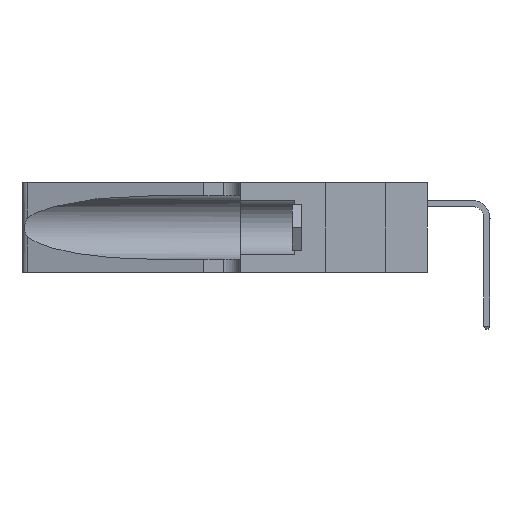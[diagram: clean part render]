
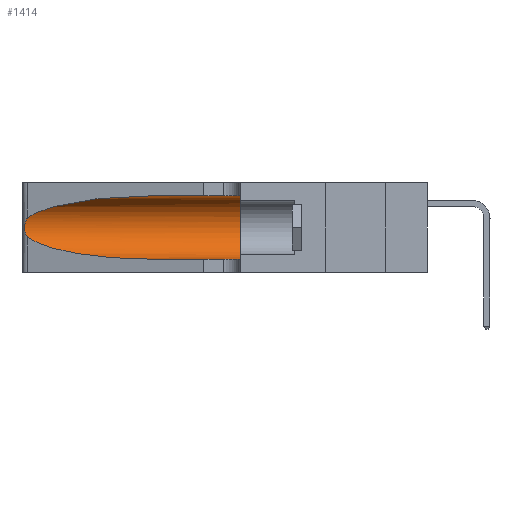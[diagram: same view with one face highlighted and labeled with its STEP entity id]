
A CAD part, left-side view. The second image highlights one B-rep face of the part: STEP entity #1414.
In plain terms, the highlighted cylindrical face has radius 3.308 mm (diameter 6.617 mm), a partial arc.
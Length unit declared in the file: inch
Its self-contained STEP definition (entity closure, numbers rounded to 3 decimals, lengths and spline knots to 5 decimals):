
#1414 = ADVANCED_FACE ( 'NONE', ( #6465 ), #5211, .F. ) ;
#1997 = LINE ( 'NONE', #23070, #11360 ) ;
#3071 = CARTESIAN_POINT ( 'NONE',  ( 0.26075, 1.23896, 0.178 ) ) ;
#3637 = ORIENTED_EDGE ( 'NONE', *, *, #45801, .T. ) ;
#5211 = CYLINDRICAL_SURFACE ( 'NONE', #36076, 0.13025 ) ;
#6465 = FACE_OUTER_BOUND ( 'NONE', #14132, .T. ) ;
#6908 = CARTESIAN_POINT ( 'NONE',  ( 0.25555, 1.22994, 0.2215 ) ) ;
#7047 = EDGE_CURVE ( 'NONE', #12578, #18360, #1997, .T. ) ;
#7082 = CARTESIAN_POINT ( 'NONE',  ( 0.25856, 1.23593, 0.16098 ) ) ;
#8322 = VERTEX_POINT ( 'NONE', #33236 ) ;
#9508 = CARTESIAN_POINT ( 'NONE',  ( 0.1305, 0.72297, 0.05475 ) ) ;
#10535 = CARTESIAN_POINT ( 'NONE',  ( 0.25487, 1.22718, 0.14631 ) ) ;
#11056 = CARTESIAN_POINT ( 'NONE',  ( 0.25639, 1.23186, 0.15144 ) ) ;
#11360 = VECTOR ( 'NONE', #50614, 39.37008 ) ;
#11673 = CARTESIAN_POINT ( 'NONE',  ( 0.1305, 0.35, 0.185 ) ) ;
#11828 = CARTESIAN_POINT ( 'NONE',  ( 0.18966, 0.96281, 0.31525 ) ) ;
#12518 = DIRECTION ( 'NONE',  ( 0., 0., -1. ) ) ;
#12578 = VERTEX_POINT ( 'NONE', #9508 ) ;
#13034 = VERTEX_POINT ( 'NONE', #43704 ) ;
#14132 = EDGE_LOOP ( 'NONE', ( #17744, #23640, #3637, #44793, #46963, #41406 ) ) ;
#14549 = CIRCLE ( 'NONE', #49179, 0.13025 ) ;
#15077 = CARTESIAN_POINT ( 'NONE',  ( 0.25487, 1.22718, 0.14631 ) ) ;
#15680 = DIRECTION ( 'NONE',  ( 0., 0., 1. ) ) ;
#17638 = VERTEX_POINT ( 'NONE', #18565 ) ;
#17744 = ORIENTED_EDGE ( 'NONE', *, *, #26415, .T. ) ;
#18306 = CARTESIAN_POINT ( 'NONE',  ( 0.1305, 1.61858, 0.31525 ) ) ;
#18360 = VERTEX_POINT ( 'NONE', #26489 ) ;
#18565 = CARTESIAN_POINT ( 'NONE',  ( 0.1305, 0.72297, 0.31525 ) ) ;
#18673 = CARTESIAN_POINT ( 'NONE',  ( 0.18966, 0.96281, 0.05475 ) ) ;
#18896 = CARTESIAN_POINT ( 'NONE',  ( 0.25639, 1.23184, 0.21858 ) ) ;
#19829 = CARTESIAN_POINT ( 'NONE',  ( 0.2373, 1.15595, 0.28018 ) ) ;
#22908 = CARTESIAN_POINT ( 'NONE',  ( 0.25854, 1.2359, 0.20912 ) ) ;
#23070 = CARTESIAN_POINT ( 'NONE',  ( 0.1305, 1.61858, 0.05475 ) ) ;
#23640 = ORIENTED_EDGE ( 'NONE', *, *, #24274, .T. ) ;
#24274 = EDGE_CURVE ( 'NONE', #8322, #31623, #50017, .T. ) ;
#25741 = VECTOR ( 'NONE', #46063, 39.37008 ) ;
#26180 = EDGE_CURVE ( 'NONE', #17638, #13034, #36244, .T. ) ;
#26415 = EDGE_CURVE ( 'NONE', #17638, #8322, #27377, .T. ) ;
#26489 = CARTESIAN_POINT ( 'NONE',  ( 0.1305, 0.35, 0.05475 ) ) ;
#26897 = CARTESIAN_POINT ( 'NONE',  ( 0.26075, 1.23896, 0.19203 ) ) ;
#27377 =( BOUNDED_CURVE ( )  B_SPLINE_CURVE ( 3, ( #39549, #11828, #19829, #47412 ),
 .UNSPECIFIED., .F., .F. ) 
 B_SPLINE_CURVE_WITH_KNOTS ( ( 4, 4 ),
 ( 1.5708, 2.84003 ),
 .UNSPECIFIED. ) 
 CURVE ( )  GEOMETRIC_REPRESENTATION_ITEM ( )  RATIONAL_B_SPLINE_CURVE ( ( 1., 0.87, 0.87, 1. ) ) 
 REPRESENTATION_ITEM ( '' )  );
#30902 = CARTESIAN_POINT ( 'NONE',  ( 0.26017, 1.23833, 0.17102 ) ) ;
#31623 = VERTEX_POINT ( 'NONE', #10535 ) ;
#32328 = CARTESIAN_POINT ( 'NONE',  ( 0.1305, 1.61858, 0.185 ) ) ;
#33236 = CARTESIAN_POINT ( 'NONE',  ( 0.25487, 1.22718, 0.22369 ) ) ;
#34856 = CARTESIAN_POINT ( 'NONE',  ( 0.25789, 1.23486, 0.15765 ) ) ;
#36076 = AXIS2_PLACEMENT_3D ( 'NONE', #32328, #36282, #12518 ) ;
#36244 = LINE ( 'NONE', #18306, #25741 ) ;
#36282 = DIRECTION ( 'NONE',  ( 0., -1., 0. ) ) ;
#36721 = EDGE_CURVE ( 'NONE', #13034, #18360, #14549, .T. ) ;
#38405 = CARTESIAN_POINT ( 'NONE',  ( 0.25487, 1.22718, 0.14631 ) ) ;
#38796 = CARTESIAN_POINT ( 'NONE',  ( 0.25555, 1.22993, 0.14849 ) ) ;
#39398 = DIRECTION ( 'NONE',  ( 0., 1., 0. ) ) ;
#39549 = CARTESIAN_POINT ( 'NONE',  ( 0.1305, 0.72297, 0.31525 ) ) ;
#39681 =( BOUNDED_CURVE ( )  B_SPLINE_CURVE ( 3, ( #38405, #42335, #18673, #46260 ),
 .UNSPECIFIED., .F., .F. ) 
 B_SPLINE_CURVE_WITH_KNOTS ( ( 4, 4 ),
 ( 3.44316, 4.71239 ),
 .UNSPECIFIED. ) 
 CURVE ( )  GEOMETRIC_REPRESENTATION_ITEM ( )  RATIONAL_B_SPLINE_CURVE ( ( 1., 0.87, 0.87, 1. ) ) 
 REPRESENTATION_ITEM ( '' )  );
#41406 = ORIENTED_EDGE ( 'NONE', *, *, #26180, .F. ) ;
#42335 = CARTESIAN_POINT ( 'NONE',  ( 0.2373, 1.15595, 0.08982 ) ) ;
#43704 = CARTESIAN_POINT ( 'NONE',  ( 0.1305, 0.35, 0.31525 ) ) ;
#44793 = ORIENTED_EDGE ( 'NONE', *, *, #7047, .T. ) ;
#45801 = EDGE_CURVE ( 'NONE', #31623, #12578, #39681, .T. ) ;
#46063 = DIRECTION ( 'NONE',  ( 0., -1., 0. ) ) ;
#46260 = CARTESIAN_POINT ( 'NONE',  ( 0.1305, 0.72297, 0.05475 ) ) ;
#46491 = CARTESIAN_POINT ( 'NONE',  ( 0.25787, 1.23484, 0.2124 ) ) ;
#46963 = ORIENTED_EDGE ( 'NONE', *, *, #36721, .F. ) ;
#47412 = CARTESIAN_POINT ( 'NONE',  ( 0.25487, 1.22718, 0.22369 ) ) ;
#49179 = AXIS2_PLACEMENT_3D ( 'NONE', #11673, #39398, #15680 ) ;
#50017 = B_SPLINE_CURVE_WITH_KNOTS ( 'NONE', 3,
 ( #50279, #6908, #18896, #46491, #22908, #50432, #26897, #3071, #30902, #7082, #34856, #11056, #38796, #15077 ),
 .UNSPECIFIED., .F., .F.,
 ( 4, 2, 2, 2, 2, 2, 4 ),
 ( 0., 0.00027, 0.00053, 0.00107, 0.0016, 0.00187, 0.00214 ),
 .UNSPECIFIED. ) ;
#50279 = CARTESIAN_POINT ( 'NONE',  ( 0.25487, 1.22718, 0.22369 ) ) ;
#50432 = CARTESIAN_POINT ( 'NONE',  ( 0.26018, 1.23835, 0.19895 ) ) ;
#50614 = DIRECTION ( 'NONE',  ( 0., -1., 0. ) ) ;
